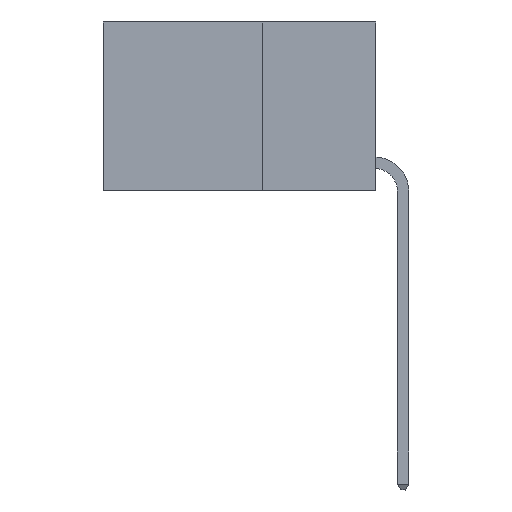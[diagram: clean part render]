
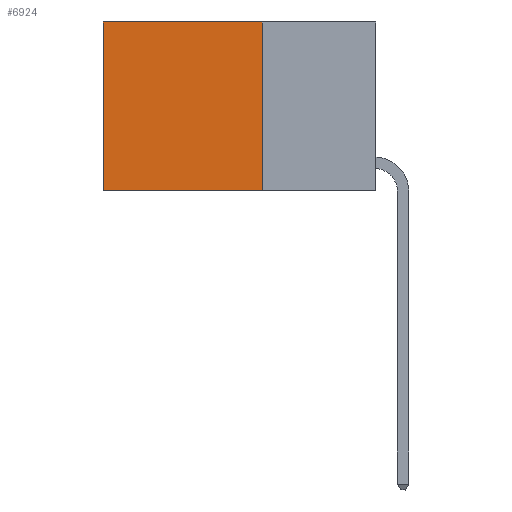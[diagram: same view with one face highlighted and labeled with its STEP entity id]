
A CAD part, left-side view. The second image highlights one B-rep face of the part: STEP entity #6924.
In plain terms, the highlighted planar face has unit normal (-1, 0, 0).
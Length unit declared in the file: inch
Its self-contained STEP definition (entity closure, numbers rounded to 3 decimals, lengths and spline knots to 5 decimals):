
#25 = EDGE_CURVE ( 'NONE', #19779, #22244, #487, .T. ) ;
#32 = LINE ( 'NONE', #5791, #19130 ) ;
#487 = LINE ( 'NONE', #11392, #4890 ) ;
#511 = EDGE_LOOP ( 'NONE', ( #11652, #1370, #2328, #3058 ) ) ;
#1370 = ORIENTED_EDGE ( 'NONE', *, *, #7115, .F. ) ;
#1542 = DIRECTION ( 'NONE',  ( 0., 0., -1. ) ) ;
#1907 = VERTEX_POINT ( 'NONE', #15618 ) ;
#2071 = CARTESIAN_POINT ( 'NONE',  ( 0.2625, 0.25, 0. ) ) ;
#2328 = ORIENTED_EDGE ( 'NONE', *, *, #13941, .F. ) ;
#3058 = ORIENTED_EDGE ( 'NONE', *, *, #25, .T. ) ;
#3908 = DIRECTION ( 'NONE',  ( 0., 1., 0. ) ) ;
#4451 = AXIS2_PLACEMENT_3D ( 'NONE', #10888, #12777, #1542 ) ;
#4890 = VECTOR ( 'NONE', #19902, 39.37008 ) ;
#5791 = CARTESIAN_POINT ( 'NONE',  ( 0.2625, 0.25, -0.37 ) ) ;
#6924 = ADVANCED_FACE ( 'NONE', ( #18311 ), #23415, .F. ) ;
#7115 = EDGE_CURVE ( 'NONE', #13308, #1907, #32, .T. ) ;
#8100 = LINE ( 'NONE', #12660, #20957 ) ;
#10888 = CARTESIAN_POINT ( 'NONE',  ( 0.2625, 0.25, 0. ) ) ;
#11392 = CARTESIAN_POINT ( 'NONE',  ( 0.2625, 0.25, 0. ) ) ;
#11652 = ORIENTED_EDGE ( 'NONE', *, *, #17727, .T. ) ;
#12659 = LINE ( 'NONE', #2071, #21082 ) ;
#12660 = CARTESIAN_POINT ( 'NONE',  ( 0.2625, 0.6, 0. ) ) ;
#12777 = DIRECTION ( 'NONE',  ( 1., 0., 0. ) ) ;
#13308 = VERTEX_POINT ( 'NONE', #18865 ) ;
#13941 = EDGE_CURVE ( 'NONE', #19779, #13308, #12659, .T. ) ;
#14478 = DIRECTION ( 'NONE',  ( 0., 0., -1. ) ) ;
#15618 = CARTESIAN_POINT ( 'NONE',  ( 0.2625, 0.6, -0.37 ) ) ;
#17727 = EDGE_CURVE ( 'NONE', #22244, #1907, #8100, .T. ) ;
#18311 = FACE_OUTER_BOUND ( 'NONE', #511, .T. ) ;
#18865 = CARTESIAN_POINT ( 'NONE',  ( 0.2625, 0.25, -0.37 ) ) ;
#19130 = VECTOR ( 'NONE', #3908, 39.37008 ) ;
#19779 = VERTEX_POINT ( 'NONE', #23070 ) ;
#19902 = DIRECTION ( 'NONE',  ( 0., 1., 0. ) ) ;
#20673 = CARTESIAN_POINT ( 'NONE',  ( 0.2625, 0.6, 0. ) ) ;
#20957 = VECTOR ( 'NONE', #14478, 39.37008 ) ;
#21082 = VECTOR ( 'NONE', #22256, 39.37008 ) ;
#22244 = VERTEX_POINT ( 'NONE', #20673 ) ;
#22256 = DIRECTION ( 'NONE',  ( 0., 0., -1. ) ) ;
#23070 = CARTESIAN_POINT ( 'NONE',  ( 0.2625, 0.25, 0. ) ) ;
#23415 = PLANE ( 'NONE',  #4451 ) ;
